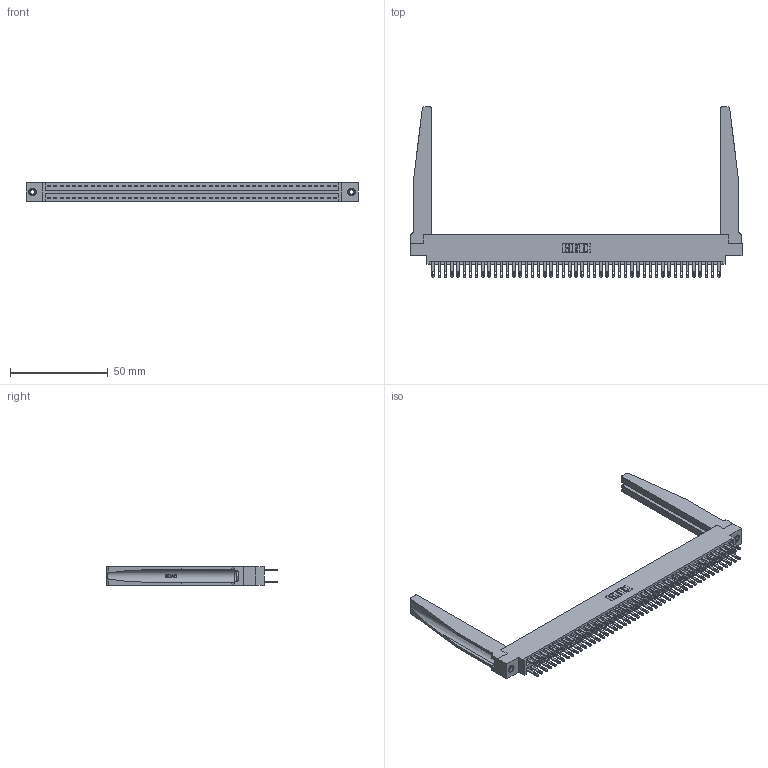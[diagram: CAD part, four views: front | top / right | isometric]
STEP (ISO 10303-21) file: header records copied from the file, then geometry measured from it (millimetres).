
FILE_DESCRIPTION (( 'STEP AP203' ), '1' );
FILE_NAME ('346-094-500-878.STEP', '2022-05-26T09:15:48', ( '' ), ( '' ), 'SwSTEP 2.0', 'SolidWorks 2020', '' );
FILE_SCHEMA (( 'CONFIG_CONTROL_DESIGN' ));
Length unit declared in the file: inch
Products named in the file (5): 346 Part_0.170 Offset - 0.156 Dia-TH; 346-220-078_345-220-078; 345-292-001_345-293-100; 345-250-001_345-250-001-102; 346-094-500-878
Assembly tree (99 placements, depth 2):
  346-094-500-878
    346 Part_0.170 Offset - 0.156 Dia-TH
    345-292-001_345-293-100  x94
    346-220-078_345-220-078  x2
    345-250-001_345-250-001-102  x2
Bounding box: 169.8 x 87.12 x 9.4 mm (x, y, z)
Volume: 23619.7 mm3; surface area: 30784.4 mm2
Topology: 99 solids, 99 shells, 4886 faces, 14803 edges, 9858 vertices
Faces by surface type: plane 2962, cylinder 1872, bspline 36, cone 12, torus 4
Entity records: 35226 total; most frequent: CARTESIAN_POINT 6741, ORIENTED_EDGE 5562, DIRECTION 4979, EDGE_CURVE 2781, VECTOR 2363, LINE 2363, VERTEX_POINT 1848, AXIS2_PLACEMENT_3D 1308
